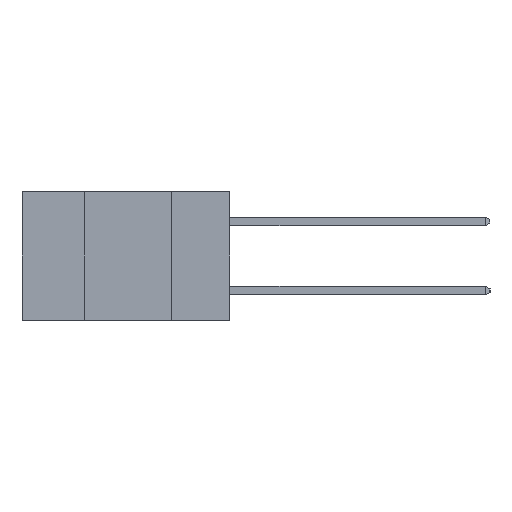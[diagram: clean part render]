
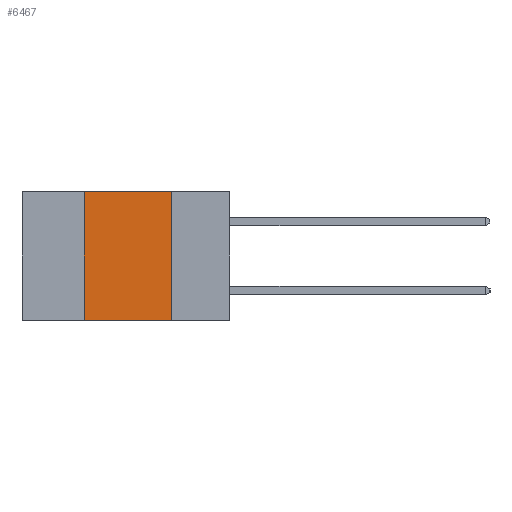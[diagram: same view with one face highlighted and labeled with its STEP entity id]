
A CAD part, left-side view. The second image highlights one B-rep face of the part: STEP entity #6467.
In plain terms, the highlighted planar face has unit normal (-1, 0, 0).
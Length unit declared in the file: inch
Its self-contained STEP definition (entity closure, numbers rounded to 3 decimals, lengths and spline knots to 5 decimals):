
#202 = VECTOR ( 'NONE', #15277, 39.37008 ) ;
#1396 = LINE ( 'NONE', #9665, #4616 ) ;
#1521 = VECTOR ( 'NONE', #15162, 39.37008 ) ;
#2467 = LINE ( 'NONE', #7558, #16286 ) ;
#3203 = CARTESIAN_POINT ( 'NONE',  ( 0., 0.6, -0.37 ) ) ;
#4616 = VECTOR ( 'NONE', #9639, 39.37008 ) ;
#5734 = EDGE_CURVE ( 'NONE', #7030, #11594, #1396, .T. ) ;
#6467 = ADVANCED_FACE ( 'NONE', ( #11119 ), #14143, .F. ) ;
#6877 = CARTESIAN_POINT ( 'NONE',  ( 0., 0.17, -0.37 ) ) ;
#7030 = VERTEX_POINT ( 'NONE', #9531 ) ;
#7277 = EDGE_CURVE ( 'NONE', #12211, #7030, #2467, .T. ) ;
#7448 = DIRECTION ( 'NONE',  ( 0., 0., 1. ) ) ;
#7558 = CARTESIAN_POINT ( 'NONE',  ( 0., 0.42, -0.37 ) ) ;
#8547 = CARTESIAN_POINT ( 'NONE',  ( 0., 0.17, 0. ) ) ;
#8692 = LINE ( 'NONE', #9785, #1521 ) ;
#9032 = ORIENTED_EDGE ( 'NONE', *, *, #10201, .F. ) ;
#9531 = CARTESIAN_POINT ( 'NONE',  ( 0., 0.42, 0. ) ) ;
#9639 = DIRECTION ( 'NONE',  ( 0., -1., 0. ) ) ;
#9665 = CARTESIAN_POINT ( 'NONE',  ( 0., 0.6, 0. ) ) ;
#9785 = CARTESIAN_POINT ( 'NONE',  ( 0., 0.17, -0.37 ) ) ;
#10056 = VERTEX_POINT ( 'NONE', #6877 ) ;
#10201 = EDGE_CURVE ( 'NONE', #11594, #10056, #8692, .T. ) ;
#10602 = ORIENTED_EDGE ( 'NONE', *, *, #7277, .F. ) ;
#10993 = LINE ( 'NONE', #3203, #202 ) ;
#11119 = FACE_OUTER_BOUND ( 'NONE', #14809, .T. ) ;
#11594 = VERTEX_POINT ( 'NONE', #8547 ) ;
#12211 = VERTEX_POINT ( 'NONE', #13803 ) ;
#13315 = ORIENTED_EDGE ( 'NONE', *, *, #17372, .T. ) ;
#13765 = AXIS2_PLACEMENT_3D ( 'NONE', #14005, #13989, #13982 ) ;
#13803 = CARTESIAN_POINT ( 'NONE',  ( 0., 0.42, -0.37 ) ) ;
#13982 = DIRECTION ( 'NONE',  ( 0., 0., -1. ) ) ;
#13989 = DIRECTION ( 'NONE',  ( 1., 0., 0. ) ) ;
#14005 = CARTESIAN_POINT ( 'NONE',  ( 0., 0.6, 0. ) ) ;
#14143 = PLANE ( 'NONE',  #13765 ) ;
#14809 = EDGE_LOOP ( 'NONE', ( #9032, #16271, #10602, #13315 ) ) ;
#15162 = DIRECTION ( 'NONE',  ( 0., 0., -1. ) ) ;
#15277 = DIRECTION ( 'NONE',  ( 0., -1., 0. ) ) ;
#16271 = ORIENTED_EDGE ( 'NONE', *, *, #5734, .F. ) ;
#16286 = VECTOR ( 'NONE', #7448, 39.37008 ) ;
#17372 = EDGE_CURVE ( 'NONE', #12211, #10056, #10993, .T. ) ;
